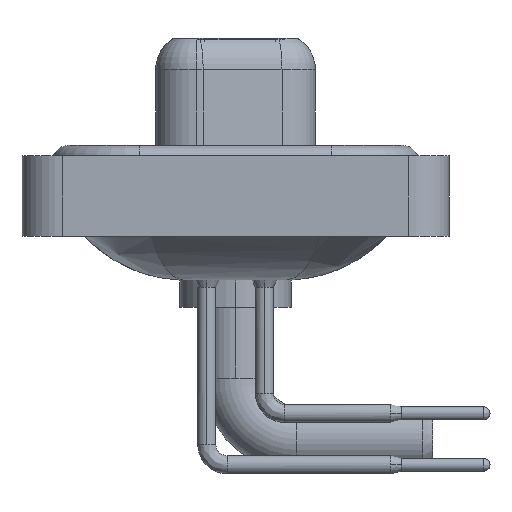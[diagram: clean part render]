
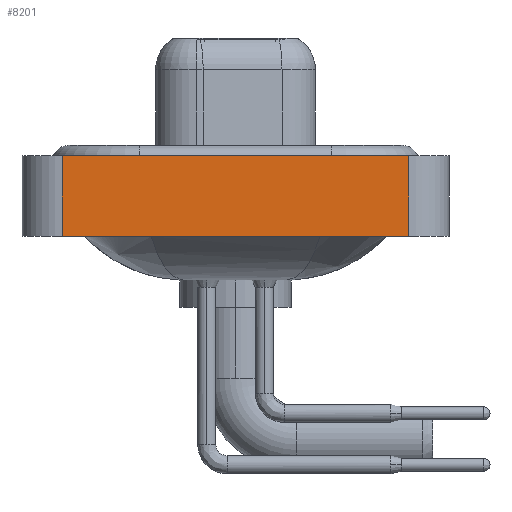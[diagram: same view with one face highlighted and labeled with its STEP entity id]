
A CAD part, left-side view. The second image highlights one B-rep face of the part: STEP entity #8201.
In plain terms, the highlighted planar face has unit normal (-1, 0, 0).
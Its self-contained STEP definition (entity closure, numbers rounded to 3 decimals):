
#1917 = CARTESIAN_POINT ( 'NONE',  ( -7.3, 8.55, -3.6 ) ) ;
#3663 = EDGE_CURVE ( 'NONE', #15079, #6383, #17363, .T. ) ;
#4047 = DIRECTION ( 'NONE',  ( 0., -1., 0. ) ) ;
#4139 = DIRECTION ( 'NONE',  ( 0., 0., 1. ) ) ;
#4320 = DIRECTION ( 'NONE',  ( 0., -1., 0. ) ) ;
#4829 = EDGE_CURVE ( 'NONE', #15079, #9631, #12832, .T. ) ;
#4937 = VECTOR ( 'NONE', #4139, 1000. ) ;
#6383 = VERTEX_POINT ( 'NONE', #15636 ) ;
#6445 = VECTOR ( 'NONE', #15198, 1000. ) ;
#7043 = ORIENTED_EDGE ( 'NONE', *, *, #13097, .F. ) ;
#7340 = DIRECTION ( 'NONE',  ( -1., 0., 0. ) ) ;
#7531 = LINE ( 'NONE', #21313, #4937 ) ;
#7829 = AXIS2_PLACEMENT_3D ( 'NONE', #19414, #7340, #21022 ) ;
#8010 = ORIENTED_EDGE ( 'NONE', *, *, #13214, .T. ) ;
#8201 = ADVANCED_FACE ( 'NONE', ( #21245 ), #15783, .T. ) ;
#8323 = ORIENTED_EDGE ( 'NONE', *, *, #3663, .F. ) ;
#9369 = CARTESIAN_POINT ( 'NONE',  ( -7.3, -8.55, -3.6 ) ) ;
#9631 = VERTEX_POINT ( 'NONE', #9369 ) ;
#11525 = VECTOR ( 'NONE', #4047, 1000. ) ;
#12498 = CARTESIAN_POINT ( 'NONE',  ( -7.3, -8.55, -3.6 ) ) ;
#12832 = LINE ( 'NONE', #12498, #11525 ) ;
#12883 = CARTESIAN_POINT ( 'NONE',  ( -7.3, -8.55, 0.4 ) ) ;
#13097 = EDGE_CURVE ( 'NONE', #6383, #14588, #14573, .T. ) ;
#13214 = EDGE_CURVE ( 'NONE', #9631, #14588, #7531, .T. ) ;
#14573 = LINE ( 'NONE', #12883, #17513 ) ;
#14588 = VERTEX_POINT ( 'NONE', #21722 ) ;
#14870 = EDGE_LOOP ( 'NONE', ( #8010, #7043, #8323, #15853 ) ) ;
#15079 = VERTEX_POINT ( 'NONE', #15788 ) ;
#15198 = DIRECTION ( 'NONE',  ( 0., 0., 1. ) ) ;
#15636 = CARTESIAN_POINT ( 'NONE',  ( -7.3, 8.55, 0.4 ) ) ;
#15783 = PLANE ( 'NONE',  #7829 ) ;
#15788 = CARTESIAN_POINT ( 'NONE',  ( -7.3, 8.55, -3.6 ) ) ;
#15853 = ORIENTED_EDGE ( 'NONE', *, *, #4829, .T. ) ;
#17363 = LINE ( 'NONE', #1917, #6445 ) ;
#17513 = VECTOR ( 'NONE', #4320, 1000. ) ;
#19414 = CARTESIAN_POINT ( 'NONE',  ( -7.3, -8.55, -3.6 ) ) ;
#21022 = DIRECTION ( 'NONE',  ( 0., 0., 1. ) ) ;
#21245 = FACE_OUTER_BOUND ( 'NONE', #14870, .T. ) ;
#21313 = CARTESIAN_POINT ( 'NONE',  ( -7.3, -8.55, -3.6 ) ) ;
#21722 = CARTESIAN_POINT ( 'NONE',  ( -7.3, -8.55, 0.4 ) ) ;
